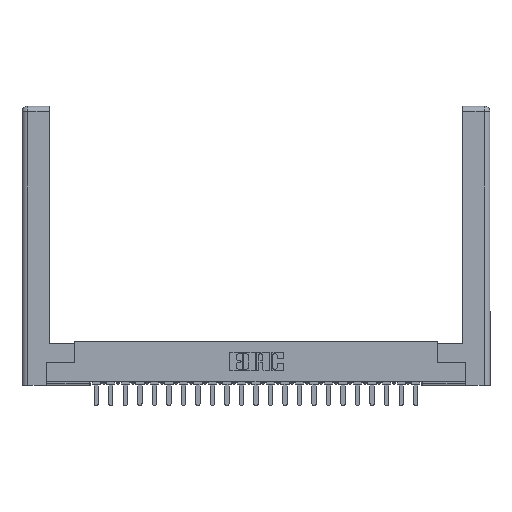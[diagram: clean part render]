
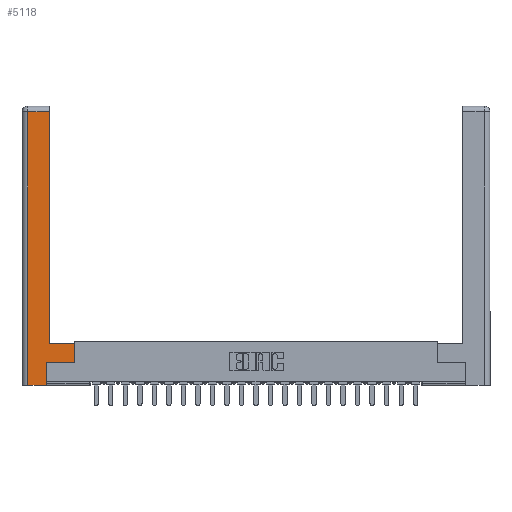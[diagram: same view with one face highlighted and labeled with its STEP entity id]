
A CAD part, top view. The second image highlights one B-rep face of the part: STEP entity #5118.
In plain terms, the highlighted planar face has unit normal (0, 0, 1).
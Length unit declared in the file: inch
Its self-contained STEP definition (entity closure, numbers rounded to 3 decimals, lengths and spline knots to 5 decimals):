
#50 = CARTESIAN_POINT ( 'NONE',  ( 0.565, 0.245, 0. ) ) ;
#347 = CARTESIAN_POINT ( 'NONE',  ( 0.0615, 0., 0. ) ) ;
#380 = DIRECTION ( 'NONE',  ( 1., 0., 0. ) ) ;
#486 = EDGE_CURVE ( 'NONE', #24250, #11216, #3539, .T. ) ;
#1048 = VERTEX_POINT ( 'NONE', #10857 ) ;
#1498 = LINE ( 'NONE', #10937, #20732 ) ;
#1593 = CARTESIAN_POINT ( 'NONE',  ( 0.565, 0.45, 0. ) ) ;
#1782 = CARTESIAN_POINT ( 'NONE',  ( 0.265, 0.245, 0. ) ) ;
#1930 = ORIENTED_EDGE ( 'NONE', *, *, #16125, .T. ) ;
#2587 = ORIENTED_EDGE ( 'NONE', *, *, #486, .T. ) ;
#3148 = DIRECTION ( 'NONE',  ( -1., 0., 0. ) ) ;
#3539 = LINE ( 'NONE', #24968, #23748 ) ;
#3617 = DIRECTION ( 'NONE',  ( 0., -1., 0. ) ) ;
#3792 = CARTESIAN_POINT ( 'NONE',  ( 0.295, 0.45, 0. ) ) ;
#3952 = LINE ( 'NONE', #7456, #24798 ) ;
#5118 = ADVANCED_FACE ( 'NONE', ( #24393 ), #6571, .F. ) ;
#5567 = VECTOR ( 'NONE', #23245, 39.37008 ) ;
#6122 = AXIS2_PLACEMENT_3D ( 'NONE', #22425, #14613, #8787 ) ;
#6571 = PLANE ( 'NONE',  #6122 ) ;
#6925 = VECTOR ( 'NONE', #13475, 39.37008 ) ;
#7256 = DIRECTION ( 'NONE',  ( -1., 0., 0. ) ) ;
#7456 = CARTESIAN_POINT ( 'NONE',  ( 0.565, 0.245, 0. ) ) ;
#8307 = LINE ( 'NONE', #1782, #5567 ) ;
#8457 = VERTEX_POINT ( 'NONE', #20042 ) ;
#8787 = DIRECTION ( 'NONE',  ( -1., 0., 0. ) ) ;
#9391 = EDGE_CURVE ( 'NONE', #18418, #8457, #20733, .T. ) ;
#9884 = CARTESIAN_POINT ( 'NONE',  ( 0.265, 0., 0. ) ) ;
#10215 = ORIENTED_EDGE ( 'NONE', *, *, #9391, .T. ) ;
#10857 = CARTESIAN_POINT ( 'NONE',  ( 0.565, 0.45, 0. ) ) ;
#10937 = CARTESIAN_POINT ( 'NONE',  ( 0.295, 0.45, 0. ) ) ;
#11216 = VERTEX_POINT ( 'NONE', #347 ) ;
#11301 = CARTESIAN_POINT ( 'NONE',  ( 0.0615, 2.94, 0. ) ) ;
#11334 = LINE ( 'NONE', #9884, #16530 ) ;
#11565 = DIRECTION ( 'NONE',  ( 1., 0., 0. ) ) ;
#12351 = ORIENTED_EDGE ( 'NONE', *, *, #17130, .T. ) ;
#12631 = CARTESIAN_POINT ( 'NONE',  ( 0.295, 3., 0. ) ) ;
#12748 = EDGE_CURVE ( 'NONE', #17027, #16853, #8307, .T. ) ;
#13475 = DIRECTION ( 'NONE',  ( 0., 1., 0. ) ) ;
#14025 = CARTESIAN_POINT ( 'NONE',  ( 0.265, 0.245, 0. ) ) ;
#14613 = DIRECTION ( 'NONE',  ( 0., 0., -1. ) ) ;
#14617 = CARTESIAN_POINT ( 'NONE',  ( 0.0615, 2.94, 0. ) ) ;
#15544 = VECTOR ( 'NONE', #16658, 39.37008 ) ;
#15893 = ORIENTED_EDGE ( 'NONE', *, *, #12748, .T. ) ;
#16102 = VERTEX_POINT ( 'NONE', #50 ) ;
#16125 = EDGE_CURVE ( 'NONE', #11216, #17027, #11334, .T. ) ;
#16333 = ORIENTED_EDGE ( 'NONE', *, *, #21522, .T. ) ;
#16415 = ORIENTED_EDGE ( 'NONE', *, *, #22363, .T. ) ;
#16530 = VECTOR ( 'NONE', #380, 39.37008 ) ;
#16658 = DIRECTION ( 'NONE',  ( 0., 1., 0. ) ) ;
#16853 = VERTEX_POINT ( 'NONE', #14025 ) ;
#17027 = VERTEX_POINT ( 'NONE', #20852 ) ;
#17069 = VECTOR ( 'NONE', #3148, 39.37008 ) ;
#17130 = EDGE_CURVE ( 'NONE', #1048, #18418, #1498, .T. ) ;
#18345 = EDGE_CURVE ( 'NONE', #16102, #1048, #18874, .T. ) ;
#18418 = VERTEX_POINT ( 'NONE', #3792 ) ;
#18874 = LINE ( 'NONE', #1593, #6925 ) ;
#19125 = ORIENTED_EDGE ( 'NONE', *, *, #18345, .T. ) ;
#20042 = CARTESIAN_POINT ( 'NONE',  ( 0.295, 2.94, 0. ) ) ;
#20410 = LINE ( 'NONE', #14617, #17069 ) ;
#20726 = EDGE_LOOP ( 'NONE', ( #10215, #16415, #2587, #1930, #15893, #16333, #19125, #12351 ) ) ;
#20732 = VECTOR ( 'NONE', #7256, 39.37008 ) ;
#20733 = LINE ( 'NONE', #12631, #15544 ) ;
#20852 = CARTESIAN_POINT ( 'NONE',  ( 0.265, 0., 0. ) ) ;
#21522 = EDGE_CURVE ( 'NONE', #16853, #16102, #3952, .T. ) ;
#22363 = EDGE_CURVE ( 'NONE', #8457, #24250, #20410, .T. ) ;
#22425 = CARTESIAN_POINT ( 'NONE',  ( 0., 0., 0. ) ) ;
#23245 = DIRECTION ( 'NONE',  ( 0., 1., 0. ) ) ;
#23748 = VECTOR ( 'NONE', #3617, 39.37008 ) ;
#24250 = VERTEX_POINT ( 'NONE', #11301 ) ;
#24393 = FACE_OUTER_BOUND ( 'NONE', #20726, .T. ) ;
#24798 = VECTOR ( 'NONE', #11565, 39.37008 ) ;
#24968 = CARTESIAN_POINT ( 'NONE',  ( 0.0615, 0., 0. ) ) ;
